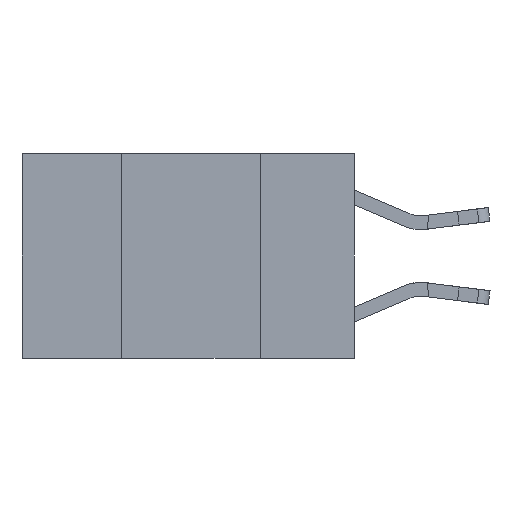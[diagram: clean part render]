
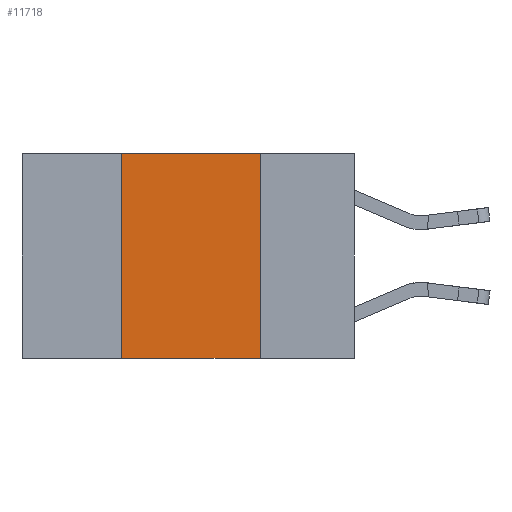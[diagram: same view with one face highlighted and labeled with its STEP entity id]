
A CAD part, left-side view. The second image highlights one B-rep face of the part: STEP entity #11718.
In plain terms, the highlighted planar face has unit normal (-1, 0, 0).
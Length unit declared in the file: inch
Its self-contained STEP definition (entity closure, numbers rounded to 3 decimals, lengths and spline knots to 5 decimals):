
#1438 = CARTESIAN_POINT ( 'NONE',  ( 0., 0.6, -0.37 ) ) ;
#1961 = PLANE ( 'NONE',  #19778 ) ;
#2127 = VECTOR ( 'NONE', #22011, 39.37008 ) ;
#2373 = VECTOR ( 'NONE', #9910, 39.37008 ) ;
#2587 = LINE ( 'NONE', #24982, #25531 ) ;
#3239 = EDGE_CURVE ( 'NONE', #16690, #26295, #2587, .T. ) ;
#4167 = EDGE_CURVE ( 'NONE', #22382, #16690, #19788, .T. ) ;
#4362 = DIRECTION ( 'NONE',  ( 0., 0., 1. ) ) ;
#8483 = ORIENTED_EDGE ( 'NONE', *, *, #19362, .T. ) ;
#8652 = VERTEX_POINT ( 'NONE', #15128 ) ;
#9225 = CARTESIAN_POINT ( 'NONE',  ( 0., 0.17, -0.37 ) ) ;
#9910 = DIRECTION ( 'NONE',  ( 0., -1., 0. ) ) ;
#10433 = DIRECTION ( 'NONE',  ( 1., 0., 0. ) ) ;
#11718 = ADVANCED_FACE ( 'NONE', ( #13053 ), #1961, .F. ) ;
#12257 = LINE ( 'NONE', #12392, #16105 ) ;
#12392 = CARTESIAN_POINT ( 'NONE',  ( 0., 0.42, 0. ) ) ;
#12640 = CARTESIAN_POINT ( 'NONE',  ( 0., 0.6, 0. ) ) ;
#13053 = FACE_OUTER_BOUND ( 'NONE', #24607, .T. ) ;
#14017 = ORIENTED_EDGE ( 'NONE', *, *, #4167, .F. ) ;
#14504 = DIRECTION ( 'NONE',  ( 0., 0., -1. ) ) ;
#15128 = CARTESIAN_POINT ( 'NONE',  ( 0., 0.42, -0.37 ) ) ;
#16105 = VECTOR ( 'NONE', #4362, 39.37008 ) ;
#16690 = VERTEX_POINT ( 'NONE', #21829 ) ;
#19362 = EDGE_CURVE ( 'NONE', #8652, #26295, #20398, .T. ) ;
#19778 = AXIS2_PLACEMENT_3D ( 'NONE', #12640, #10433, #27203 ) ;
#19788 = LINE ( 'NONE', #24198, #2127 ) ;
#20398 = LINE ( 'NONE', #1438, #2373 ) ;
#21192 = ORIENTED_EDGE ( 'NONE', *, *, #3239, .F. ) ;
#21829 = CARTESIAN_POINT ( 'NONE',  ( 0., 0.17, 0. ) ) ;
#22011 = DIRECTION ( 'NONE',  ( 0., -1., 0. ) ) ;
#22382 = VERTEX_POINT ( 'NONE', #23860 ) ;
#22606 = EDGE_CURVE ( 'NONE', #8652, #22382, #12257, .T. ) ;
#23335 = ORIENTED_EDGE ( 'NONE', *, *, #22606, .F. ) ;
#23860 = CARTESIAN_POINT ( 'NONE',  ( 0., 0.42, 0. ) ) ;
#24198 = CARTESIAN_POINT ( 'NONE',  ( 0., 0.6, 0. ) ) ;
#24607 = EDGE_LOOP ( 'NONE', ( #21192, #14017, #23335, #8483 ) ) ;
#24982 = CARTESIAN_POINT ( 'NONE',  ( 0., 0.17, 0. ) ) ;
#25531 = VECTOR ( 'NONE', #14504, 39.37008 ) ;
#26295 = VERTEX_POINT ( 'NONE', #9225 ) ;
#27203 = DIRECTION ( 'NONE',  ( 0., 0., -1. ) ) ;
